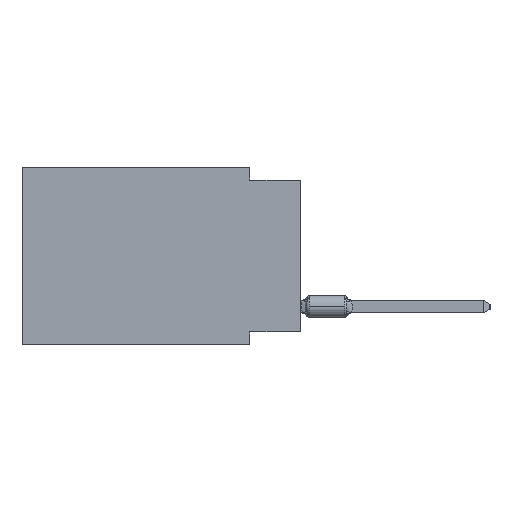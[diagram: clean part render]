
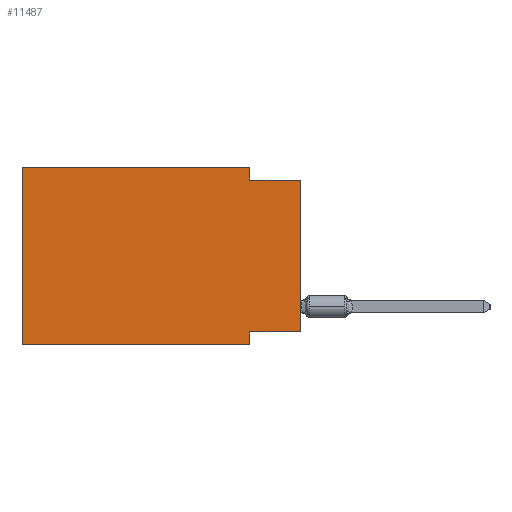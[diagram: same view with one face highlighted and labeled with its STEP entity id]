
A CAD part, left-side view. The second image highlights one B-rep face of the part: STEP entity #11487.
In plain terms, the highlighted planar face has unit normal (-1, 0, 0).
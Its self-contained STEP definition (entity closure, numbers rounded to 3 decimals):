
#577 = DIRECTION ( 'NONE',  ( 0., 0., -1. ) ) ;
#768 = EDGE_CURVE ( 'NONE', #17493, #33029, #23751, .T. ) ;
#1191 = EDGE_CURVE ( 'NONE', #18379, #13307, #11796, .T. ) ;
#3383 = EDGE_LOOP ( 'NONE', ( #19786, #5102, #30293, #3613, #25262, #28477, #14946, #22952 ) ) ;
#3613 = ORIENTED_EDGE ( 'NONE', *, *, #23942, .F. ) ;
#4852 = CARTESIAN_POINT ( 'NONE',  ( 0., 0., -8.255 ) ) ;
#5102 = ORIENTED_EDGE ( 'NONE', *, *, #8379, .F. ) ;
#5354 = VECTOR ( 'NONE', #33075, 1000. ) ;
#5682 = DIRECTION ( 'NONE',  ( 0., 0., -1. ) ) ;
#5820 = CARTESIAN_POINT ( 'NONE',  ( 0., 13.97, 0. ) ) ;
#8379 = EDGE_CURVE ( 'NONE', #29018, #26415, #8762, .T. ) ;
#8746 = LINE ( 'NONE', #23997, #18011 ) ;
#8762 = LINE ( 'NONE', #24516, #27592 ) ;
#8982 = LINE ( 'NONE', #11861, #9492 ) ;
#9492 = VECTOR ( 'NONE', #22191, 1000. ) ;
#10813 = LINE ( 'NONE', #18258, #30127 ) ;
#11487 = ADVANCED_FACE ( 'NONE', ( #26227 ), #16211, .F. ) ;
#11796 = LINE ( 'NONE', #29761, #21791 ) ;
#11861 = CARTESIAN_POINT ( 'NONE',  ( 0., 0., 0. ) ) ;
#12289 = EDGE_CURVE ( 'NONE', #14556, #29018, #8746, .T. ) ;
#12915 = CARTESIAN_POINT ( 'NONE',  ( 0., 13.97, -8.89 ) ) ;
#13307 = VERTEX_POINT ( 'NONE', #25709 ) ;
#14556 = VERTEX_POINT ( 'NONE', #29988 ) ;
#14903 = EDGE_CURVE ( 'NONE', #24585, #18379, #10813, .T. ) ;
#14946 = ORIENTED_EDGE ( 'NONE', *, *, #1191, .F. ) ;
#15947 = CARTESIAN_POINT ( 'NONE',  ( 0., 13.97, 0. ) ) ;
#16181 = DIRECTION ( 'NONE',  ( 0., -1., 0. ) ) ;
#16211 = PLANE ( 'NONE',  #22852 ) ;
#17493 = VERTEX_POINT ( 'NONE', #22278 ) ;
#17968 = VECTOR ( 'NONE', #18664, 1000. ) ;
#18011 = VECTOR ( 'NONE', #577, 1000. ) ;
#18258 = CARTESIAN_POINT ( 'NONE',  ( 0., 0., -8.255 ) ) ;
#18379 = VERTEX_POINT ( 'NONE', #21706 ) ;
#18439 = EDGE_CURVE ( 'NONE', #24585, #26415, #8982, .T. ) ;
#18664 = DIRECTION ( 'NONE',  ( 0., 0., 1. ) ) ;
#19632 = CARTESIAN_POINT ( 'NONE',  ( 0., 2.54, -0.635 ) ) ;
#19786 = ORIENTED_EDGE ( 'NONE', *, *, #18439, .T. ) ;
#20716 = LINE ( 'NONE', #12915, #5354 ) ;
#21344 = EDGE_CURVE ( 'NONE', #17493, #13307, #20716, .T. ) ;
#21479 = CARTESIAN_POINT ( 'NONE',  ( 0., 13.97, 0. ) ) ;
#21706 = CARTESIAN_POINT ( 'NONE',  ( 0., 2.54, -8.255 ) ) ;
#21791 = VECTOR ( 'NONE', #31957, 1000. ) ;
#22191 = DIRECTION ( 'NONE',  ( 0., 0., 1. ) ) ;
#22278 = CARTESIAN_POINT ( 'NONE',  ( 0., 13.97, -8.89 ) ) ;
#22852 = AXIS2_PLACEMENT_3D ( 'NONE', #21479, #26738, #5682 ) ;
#22952 = ORIENTED_EDGE ( 'NONE', *, *, #14903, .F. ) ;
#23471 = LINE ( 'NONE', #5820, #24458 ) ;
#23526 = DIRECTION ( 'NONE',  ( 0., 1., 0. ) ) ;
#23751 = LINE ( 'NONE', #15947, #17968 ) ;
#23942 = EDGE_CURVE ( 'NONE', #33029, #14556, #23471, .T. ) ;
#23997 = CARTESIAN_POINT ( 'NONE',  ( 0., 2.54, 0. ) ) ;
#24458 = VECTOR ( 'NONE', #16181, 1000. ) ;
#24516 = CARTESIAN_POINT ( 'NONE',  ( 0., 0., -0.635 ) ) ;
#24585 = VERTEX_POINT ( 'NONE', #4852 ) ;
#24598 = CARTESIAN_POINT ( 'NONE',  ( 0., 0., -0.635 ) ) ;
#25262 = ORIENTED_EDGE ( 'NONE', *, *, #768, .F. ) ;
#25709 = CARTESIAN_POINT ( 'NONE',  ( 0., 2.54, -8.89 ) ) ;
#26227 = FACE_OUTER_BOUND ( 'NONE', #3383, .T. ) ;
#26415 = VERTEX_POINT ( 'NONE', #24598 ) ;
#26738 = DIRECTION ( 'NONE',  ( 1., 0., 0. ) ) ;
#27592 = VECTOR ( 'NONE', #31807, 1000. ) ;
#28477 = ORIENTED_EDGE ( 'NONE', *, *, #21344, .T. ) ;
#28829 = CARTESIAN_POINT ( 'NONE',  ( 0., 13.97, 0. ) ) ;
#29018 = VERTEX_POINT ( 'NONE', #19632 ) ;
#29761 = CARTESIAN_POINT ( 'NONE',  ( 0., 2.54, -8.89 ) ) ;
#29988 = CARTESIAN_POINT ( 'NONE',  ( 0., 2.54, 0. ) ) ;
#30127 = VECTOR ( 'NONE', #23526, 1000. ) ;
#30293 = ORIENTED_EDGE ( 'NONE', *, *, #12289, .F. ) ;
#31807 = DIRECTION ( 'NONE',  ( 0., -1., 0. ) ) ;
#31957 = DIRECTION ( 'NONE',  ( 0., 0., -1. ) ) ;
#33029 = VERTEX_POINT ( 'NONE', #28829 ) ;
#33075 = DIRECTION ( 'NONE',  ( 0., -1., 0. ) ) ;
